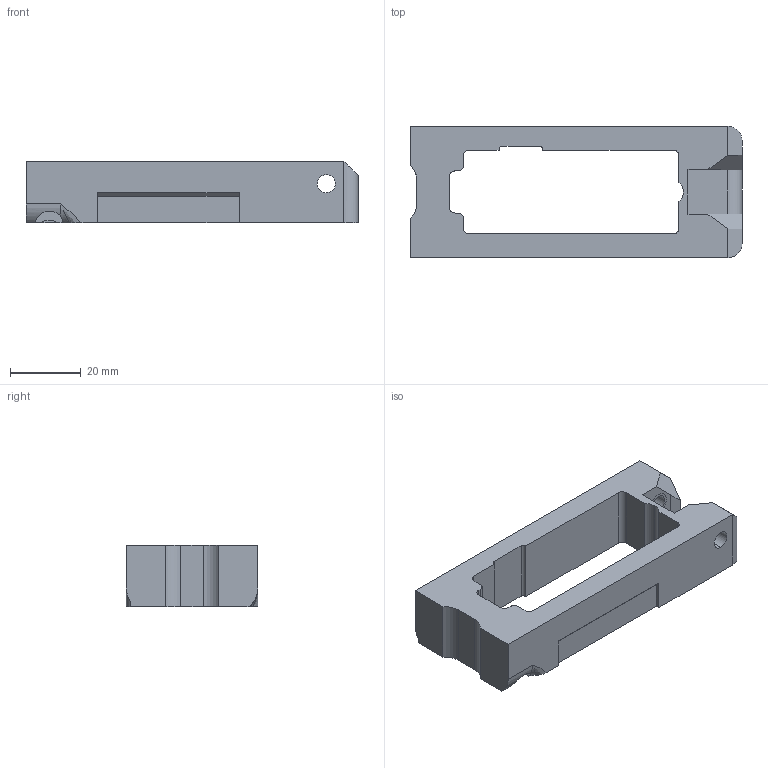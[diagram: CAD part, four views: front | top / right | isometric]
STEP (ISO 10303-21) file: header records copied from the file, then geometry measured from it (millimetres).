
FILE_DESCRIPTION (( 'STEP AP214' ), '1' );
FILE_NAME ('Magwell_1_1_Modified.step', '2019-12-18T03:08:09', ( '' ), ( '' ), 'SwSTEP 2.0', 'SolidWorks 2019', '' );
FILE_SCHEMA (( 'AUTOMOTIVE_DESIGN' ));
Length unit declared in the file: millimetre
Products named in the file (1): Magwell_1_1_Modified
Bounding box: 93.83 x 37.13 x 17.46 mm (x, y, z)
Volume: 29654.4 mm3; surface area: 12224.8 mm2
Topology: 2 solids, 2 shells, 106 faces, 320 edges, 208 vertices
Faces by surface type: plane 49, cylinder 33, sphere 22, bspline 1, torus 1
Entity records: 3449 total; most frequent: CARTESIAN_POINT 702, DIRECTION 585, ORIENTED_EDGE 550, EDGE_CURVE 275, AXIS2_PLACEMENT_3D 216, VERTEX_POINT 186, LINE 153, VECTOR 153
